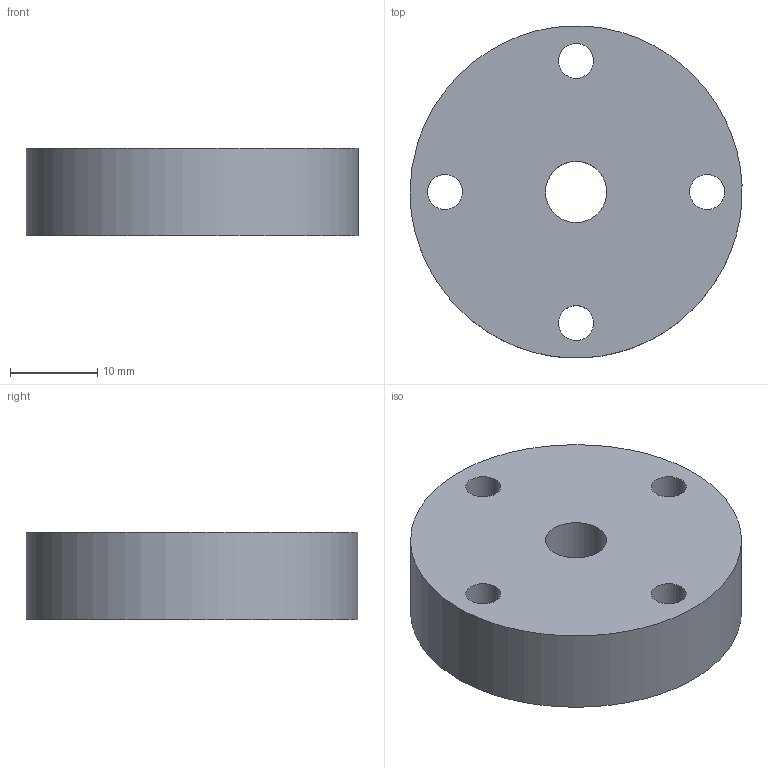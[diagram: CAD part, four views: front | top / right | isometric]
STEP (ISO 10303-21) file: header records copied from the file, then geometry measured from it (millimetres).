
FILE_DESCRIPTION(/* description */ (''),/* implementation_level */ '2;1');
FILE_NAME(/* name */ 'HiLo JIG_drill guide 7mm v1.step',/* time_stamp */ '2022-08-27T22:33:33-04:00',/* author */ (''),/* organization */ (''),/* preprocessor_version */ 'ST-DEVELOPER v19',/* originating_system */ 'Autodesk Translation Framework v11.7.0.108',/* authorisation */ '');
FILE_SCHEMA (('AUTOMOTIVE_DESIGN { 1 0 10303 214 3 1 1 }'));
Length unit declared in the file: millimetre
Products named in the file (1): HiLo JIG_drill guide 7mm
Bounding box: 37.98 x 37.96 x 10 mm (x, y, z)
Volume: 10370 mm3; surface area: 4163.1 mm2
Topology: 1 solids, 1 shells, 174 faces, 489 edges, 326 vertices
Faces by surface type: bspline 115, plane 54, cylinder 5
Full cylindrical faces by diameter (mm): 4 x4, 7 x1
Entity records: 6783 total; most frequent: CARTESIAN_POINT 3025, ORIENTED_EDGE 978, EDGE_CURVE 489, DIRECTION 389, VERTEX_POINT 326, LINE 249, VECTOR 249, B_SPLINE_CURVE_WITH_KNOTS 228
